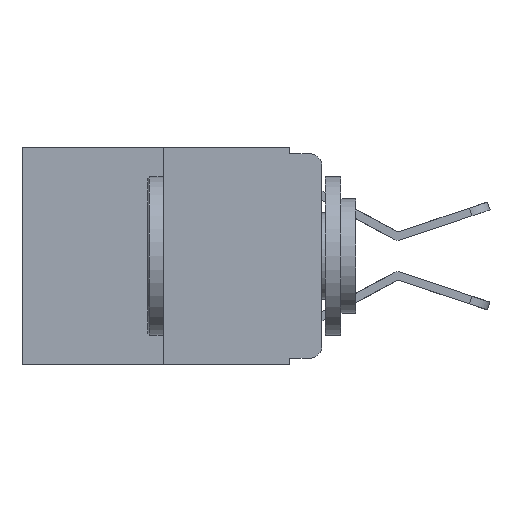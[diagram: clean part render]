
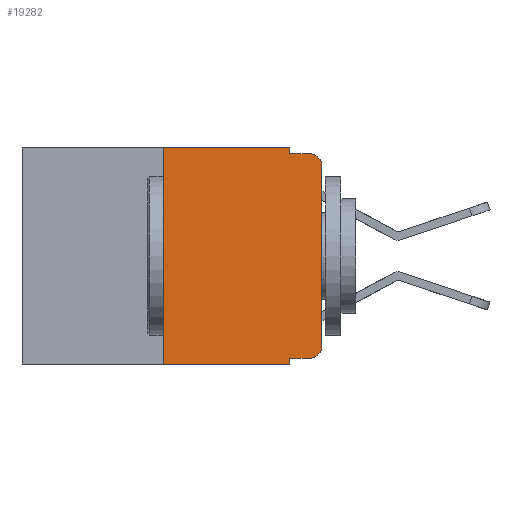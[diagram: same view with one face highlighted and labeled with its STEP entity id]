
A CAD part, left-side view. The second image highlights one B-rep face of the part: STEP entity #19282.
In plain terms, the highlighted planar face has unit normal (-1, 0, 0).
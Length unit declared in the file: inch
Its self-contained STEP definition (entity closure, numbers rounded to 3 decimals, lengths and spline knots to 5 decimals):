
#277 = LINE ( 'NONE', #11128, #21734 ) ;
#533 = ORIENTED_EDGE ( 'NONE', *, *, #13335, .F. ) ;
#778 = VERTEX_POINT ( 'NONE', #6231 ) ;
#982 = ORIENTED_EDGE ( 'NONE', *, *, #10049, .T. ) ;
#1768 = VERTEX_POINT ( 'NONE', #8297 ) ;
#1808 = VECTOR ( 'NONE', #12718, 39.37008 ) ;
#2021 = VECTOR ( 'NONE', #23464, 39.37008 ) ;
#2339 = EDGE_CURVE ( 'NONE', #14619, #17338, #13928, .T. ) ;
#2724 = LINE ( 'NONE', #10239, #9822 ) ;
#2802 = VECTOR ( 'NONE', #18565, 39.37008 ) ;
#2900 = CARTESIAN_POINT ( 'NONE',  ( 0., 0.473, -0.343 ) ) ;
#4404 = VERTEX_POINT ( 'NONE', #20066 ) ;
#4579 = VERTEX_POINT ( 'NONE', #9672 ) ;
#4615 = DIRECTION ( 'NONE',  ( 0., 0., -1. ) ) ;
#4625 = VERTEX_POINT ( 'NONE', #17081 ) ;
#5813 = DIRECTION ( 'NONE',  ( 0., -1., 0. ) ) ;
#6231 = CARTESIAN_POINT ( 'NONE',  ( 0., 0., -0.313 ) ) ;
#6703 = LINE ( 'NONE', #8436, #14095 ) ;
#6738 = FACE_OUTER_BOUND ( 'NONE', #16225, .T. ) ;
#6830 = CARTESIAN_POINT ( 'NONE',  ( 0., 0.051, -0.01 ) ) ;
#7417 = VECTOR ( 'NONE', #18564, 39.37008 ) ;
#7965 = CIRCLE ( 'NONE', #11882, 0.02 ) ;
#8297 = CARTESIAN_POINT ( 'NONE',  ( 0., 0.02, -0.333 ) ) ;
#8436 = CARTESIAN_POINT ( 'NONE',  ( 0., 0.473, 0. ) ) ;
#9158 = LINE ( 'NONE', #24244, #1808 ) ;
#9672 = CARTESIAN_POINT ( 'NONE',  ( 0., 0.051, -0.343 ) ) ;
#9822 = VECTOR ( 'NONE', #10363, 39.37008 ) ;
#10049 = EDGE_CURVE ( 'NONE', #4404, #17338, #15528, .T. ) ;
#10239 = CARTESIAN_POINT ( 'NONE',  ( 0., 0.051, 0. ) ) ;
#10310 = PLANE ( 'NONE',  #21715 ) ;
#10363 = DIRECTION ( 'NONE',  ( 0., 0., -1. ) ) ;
#10419 = ORIENTED_EDGE ( 'NONE', *, *, #21658, .T. ) ;
#10530 = DIRECTION ( 'NONE',  ( -1., 0., 0. ) ) ;
#11076 = VECTOR ( 'NONE', #19939, 39.37008 ) ;
#11128 = CARTESIAN_POINT ( 'NONE',  ( 0., 0.051, -0.333 ) ) ;
#11477 = EDGE_CURVE ( 'NONE', #15125, #17191, #9158, .T. ) ;
#11882 = AXIS2_PLACEMENT_3D ( 'NONE', #23373, #12579, #21518 ) ;
#12088 = CARTESIAN_POINT ( 'NONE',  ( 0., 0.25, -0.343 ) ) ;
#12263 = ORIENTED_EDGE ( 'NONE', *, *, #11477, .F. ) ;
#12492 = ORIENTED_EDGE ( 'NONE', *, *, #19429, .F. ) ;
#12503 = CARTESIAN_POINT ( 'NONE',  ( 0., 0.473, 0. ) ) ;
#12579 = DIRECTION ( 'NONE',  ( -1., 0., 0. ) ) ;
#12718 = DIRECTION ( 'NONE',  ( 0., 0., 1. ) ) ;
#12859 = CARTESIAN_POINT ( 'NONE',  ( 0., 0.051, 0. ) ) ;
#12982 = LINE ( 'NONE', #14613, #7417 ) ;
#13335 = EDGE_CURVE ( 'NONE', #17191, #4625, #6703, .T. ) ;
#13928 = LINE ( 'NONE', #16275, #2021 ) ;
#14064 = ORIENTED_EDGE ( 'NONE', *, *, #2339, .F. ) ;
#14095 = VECTOR ( 'NONE', #17944, 39.37008 ) ;
#14286 = EDGE_CURVE ( 'NONE', #778, #4404, #12982, .T. ) ;
#14613 = CARTESIAN_POINT ( 'NONE',  ( 0., 0., 0. ) ) ;
#14619 = VERTEX_POINT ( 'NONE', #6830 ) ;
#14853 = LINE ( 'NONE', #12859, #2802 ) ;
#15125 = VERTEX_POINT ( 'NONE', #12088 ) ;
#15528 = CIRCLE ( 'NONE', #16336, 0.02 ) ;
#16225 = EDGE_LOOP ( 'NONE', ( #17647, #982, #14064, #24177, #533, #12263, #10419, #12492, #21349, #23125 ) ) ;
#16275 = CARTESIAN_POINT ( 'NONE',  ( 0., 0.051, -0.01 ) ) ;
#16336 = AXIS2_PLACEMENT_3D ( 'NONE', #19810, #10530, #4615 ) ;
#16350 = DIRECTION ( 'NONE',  ( 1., 0., 0. ) ) ;
#16440 = EDGE_CURVE ( 'NONE', #19296, #1768, #277, .T. ) ;
#17081 = CARTESIAN_POINT ( 'NONE',  ( 0., 0.051, 0. ) ) ;
#17191 = VERTEX_POINT ( 'NONE', #20734 ) ;
#17338 = VERTEX_POINT ( 'NONE', #17756 ) ;
#17647 = ORIENTED_EDGE ( 'NONE', *, *, #14286, .T. ) ;
#17756 = CARTESIAN_POINT ( 'NONE',  ( 0., 0.02, -0.01 ) ) ;
#17944 = DIRECTION ( 'NONE',  ( 0., -1., 0. ) ) ;
#18093 = CARTESIAN_POINT ( 'NONE',  ( 0., 0.051, -0.333 ) ) ;
#18201 = LINE ( 'NONE', #2900, #11076 ) ;
#18280 = EDGE_CURVE ( 'NONE', #4625, #14619, #2724, .T. ) ;
#18564 = DIRECTION ( 'NONE',  ( 0., 0., 1. ) ) ;
#18565 = DIRECTION ( 'NONE',  ( 0., 0., -1. ) ) ;
#19282 = ADVANCED_FACE ( 'NONE', ( #6738 ), #10310, .F. ) ;
#19296 = VERTEX_POINT ( 'NONE', #18093 ) ;
#19429 = EDGE_CURVE ( 'NONE', #19296, #4579, #14853, .T. ) ;
#19810 = CARTESIAN_POINT ( 'NONE',  ( 0., 0.02, -0.03 ) ) ;
#19939 = DIRECTION ( 'NONE',  ( 0., -1., 0. ) ) ;
#19952 = DIRECTION ( 'NONE',  ( 0., 0., -1. ) ) ;
#20066 = CARTESIAN_POINT ( 'NONE',  ( 0., 0., -0.03 ) ) ;
#20734 = CARTESIAN_POINT ( 'NONE',  ( 0., 0.25, 0. ) ) ;
#21349 = ORIENTED_EDGE ( 'NONE', *, *, #16440, .T. ) ;
#21518 = DIRECTION ( 'NONE',  ( 0., 0., -1. ) ) ;
#21658 = EDGE_CURVE ( 'NONE', #15125, #4579, #18201, .T. ) ;
#21715 = AXIS2_PLACEMENT_3D ( 'NONE', #12503, #16350, #19952 ) ;
#21734 = VECTOR ( 'NONE', #5813, 39.37008 ) ;
#22050 = EDGE_CURVE ( 'NONE', #1768, #778, #7965, .T. ) ;
#23125 = ORIENTED_EDGE ( 'NONE', *, *, #22050, .T. ) ;
#23373 = CARTESIAN_POINT ( 'NONE',  ( 0., 0.02, -0.313 ) ) ;
#23464 = DIRECTION ( 'NONE',  ( 0., -1., 0. ) ) ;
#24177 = ORIENTED_EDGE ( 'NONE', *, *, #18280, .F. ) ;
#24244 = CARTESIAN_POINT ( 'NONE',  ( 0., 0.25, 0. ) ) ;
